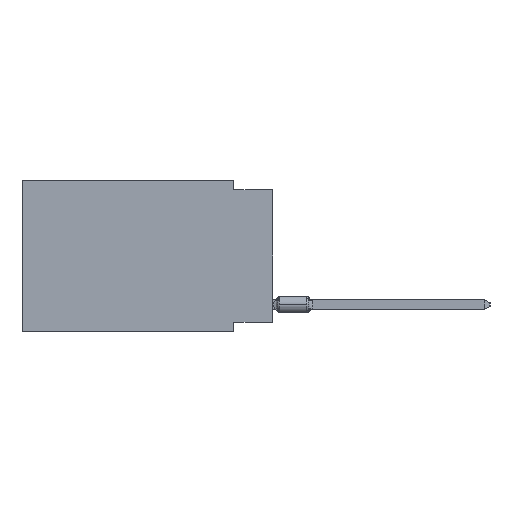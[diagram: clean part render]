
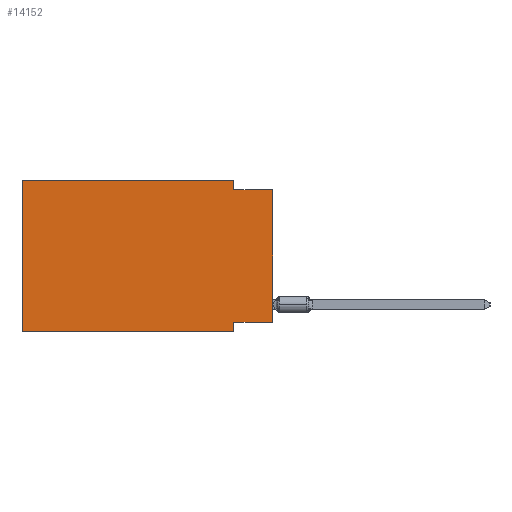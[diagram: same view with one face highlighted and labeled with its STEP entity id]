
A CAD part, left-side view. The second image highlights one B-rep face of the part: STEP entity #14152.
In plain terms, the highlighted planar face has unit normal (-1, 0, 0).
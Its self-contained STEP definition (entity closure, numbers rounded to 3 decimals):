
#1285 = VECTOR ( 'NONE', #17490, 1000. ) ;
#2223 = ORIENTED_EDGE ( 'NONE', *, *, #35261, .F. ) ;
#3593 = PLANE ( 'NONE',  #22511 ) ;
#5868 = DIRECTION ( 'NONE',  ( 0., 1., 0. ) ) ;
#6841 = CARTESIAN_POINT ( 'NONE',  ( 0., 2.54, 0. ) ) ;
#9559 = ORIENTED_EDGE ( 'NONE', *, *, #40760, .F. ) ;
#10066 = LINE ( 'NONE', #45612, #10491 ) ;
#10491 = VECTOR ( 'NONE', #56877, 1000. ) ;
#10519 = ORIENTED_EDGE ( 'NONE', *, *, #62685, .F. ) ;
#12064 = EDGE_LOOP ( 'NONE', ( #45824, #41005, #19277, #27933, #2223, #61620, #9559, #10519 ) ) ;
#14152 = ADVANCED_FACE ( 'NONE', ( #50433 ), #3593, .F. ) ;
#15140 = VERTEX_POINT ( 'NONE', #47379 ) ;
#15566 = VECTOR ( 'NONE', #50112, 1000. ) ;
#16743 = CARTESIAN_POINT ( 'NONE',  ( 0., 0., -0.635 ) ) ;
#17403 = CARTESIAN_POINT ( 'NONE',  ( 0., 2.54, 0. ) ) ;
#17490 = DIRECTION ( 'NONE',  ( 0., 0., 1. ) ) ;
#18804 = CARTESIAN_POINT ( 'NONE',  ( 0., 0., -9.271 ) ) ;
#19277 = ORIENTED_EDGE ( 'NONE', *, *, #36197, .F. ) ;
#19667 = LINE ( 'NONE', #50439, #15566 ) ;
#22511 = AXIS2_PLACEMENT_3D ( 'NONE', #55873, #34699, #50758 ) ;
#22516 = CARTESIAN_POINT ( 'NONE',  ( 0., 16.383, 0. ) ) ;
#25849 = VECTOR ( 'NONE', #5868, 1000. ) ;
#27634 = LINE ( 'NONE', #22516, #51113 ) ;
#27933 = ORIENTED_EDGE ( 'NONE', *, *, #64272, .F. ) ;
#28071 = VERTEX_POINT ( 'NONE', #38156 ) ;
#30522 = VERTEX_POINT ( 'NONE', #16743 ) ;
#32547 = LINE ( 'NONE', #63298, #65042 ) ;
#32879 = LINE ( 'NONE', #38663, #1285 ) ;
#34699 = DIRECTION ( 'NONE',  ( 1., 0., 0. ) ) ;
#35261 = EDGE_CURVE ( 'NONE', #15140, #35653, #19667, .T. ) ;
#35653 = VERTEX_POINT ( 'NONE', #41090 ) ;
#35742 = EDGE_CURVE ( 'NONE', #66599, #30522, #32879, .T. ) ;
#36197 = EDGE_CURVE ( 'NONE', #53646, #59832, #58423, .T. ) ;
#36957 = LINE ( 'NONE', #57790, #25849 ) ;
#37387 = VECTOR ( 'NONE', #48171, 1000. ) ;
#37399 = EDGE_CURVE ( 'NONE', #59832, #30522, #48182, .T. ) ;
#38156 = CARTESIAN_POINT ( 'NONE',  ( 0., 2.54, -9.906 ) ) ;
#38221 = DIRECTION ( 'NONE',  ( 0., -1., 0. ) ) ;
#38663 = CARTESIAN_POINT ( 'NONE',  ( 0., 0., 0. ) ) ;
#39230 = EDGE_CURVE ( 'NONE', #15140, #28071, #32547, .T. ) ;
#40491 = CARTESIAN_POINT ( 'NONE',  ( 0., 2.54, -0.635 ) ) ;
#40760 = EDGE_CURVE ( 'NONE', #45837, #28071, #10066, .T. ) ;
#41005 = ORIENTED_EDGE ( 'NONE', *, *, #37399, .F. ) ;
#41090 = CARTESIAN_POINT ( 'NONE',  ( 0., 16.383, 0. ) ) ;
#45089 = VECTOR ( 'NONE', #52976, 1000. ) ;
#45612 = CARTESIAN_POINT ( 'NONE',  ( 0., 2.54, -9.906 ) ) ;
#45824 = ORIENTED_EDGE ( 'NONE', *, *, #35742, .T. ) ;
#45837 = VERTEX_POINT ( 'NONE', #67011 ) ;
#47379 = CARTESIAN_POINT ( 'NONE',  ( 0., 16.383, -9.906 ) ) ;
#47514 = CARTESIAN_POINT ( 'NONE',  ( 0., 0., -0.635 ) ) ;
#48171 = DIRECTION ( 'NONE',  ( 0., 0., -1. ) ) ;
#48182 = LINE ( 'NONE', #47514, #45089 ) ;
#50112 = DIRECTION ( 'NONE',  ( 0., 0., 1. ) ) ;
#50433 = FACE_OUTER_BOUND ( 'NONE', #12064, .T. ) ;
#50439 = CARTESIAN_POINT ( 'NONE',  ( 0., 16.383, 0. ) ) ;
#50758 = DIRECTION ( 'NONE',  ( 0., 0., -1. ) ) ;
#51113 = VECTOR ( 'NONE', #38221, 1000. ) ;
#52976 = DIRECTION ( 'NONE',  ( 0., -1., 0. ) ) ;
#53646 = VERTEX_POINT ( 'NONE', #6841 ) ;
#55873 = CARTESIAN_POINT ( 'NONE',  ( 0., 16.383, 0. ) ) ;
#56877 = DIRECTION ( 'NONE',  ( 0., 0., -1. ) ) ;
#57790 = CARTESIAN_POINT ( 'NONE',  ( 0., 0., -9.271 ) ) ;
#58423 = LINE ( 'NONE', #17403, #37387 ) ;
#58850 = DIRECTION ( 'NONE',  ( 0., -1., 0. ) ) ;
#59832 = VERTEX_POINT ( 'NONE', #40491 ) ;
#61620 = ORIENTED_EDGE ( 'NONE', *, *, #39230, .T. ) ;
#62685 = EDGE_CURVE ( 'NONE', #66599, #45837, #36957, .T. ) ;
#63298 = CARTESIAN_POINT ( 'NONE',  ( 0., 16.383, -9.906 ) ) ;
#64272 = EDGE_CURVE ( 'NONE', #35653, #53646, #27634, .T. ) ;
#65042 = VECTOR ( 'NONE', #58850, 1000. ) ;
#66599 = VERTEX_POINT ( 'NONE', #18804 ) ;
#67011 = CARTESIAN_POINT ( 'NONE',  ( 0., 2.54, -9.271 ) ) ;
